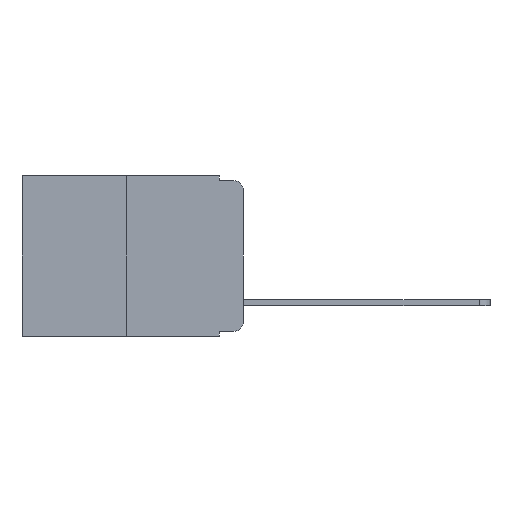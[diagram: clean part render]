
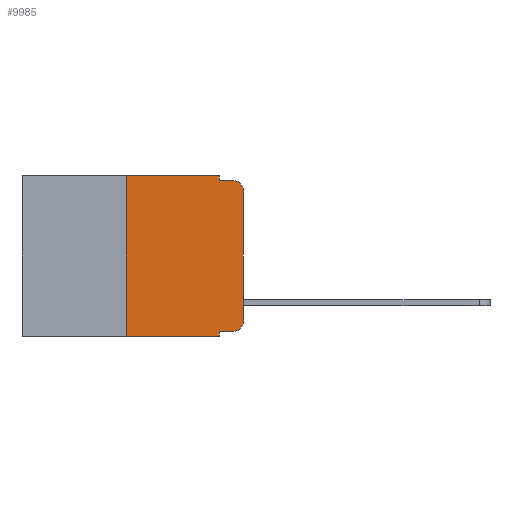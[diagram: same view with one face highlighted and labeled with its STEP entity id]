
A CAD part, left-side view. The second image highlights one B-rep face of the part: STEP entity #9985.
In plain terms, the highlighted planar face has unit normal (-1, 0, 0).
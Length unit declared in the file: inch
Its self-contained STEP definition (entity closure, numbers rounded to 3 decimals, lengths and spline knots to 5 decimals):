
#44 = EDGE_CURVE ( 'NONE', #7193, #5768, #9298, .T. ) ;
#143 = DIRECTION ( 'NONE',  ( 0., 0., -1. ) ) ;
#144 = DIRECTION ( 'NONE',  ( 1., 0., 0. ) ) ;
#146 = CARTESIAN_POINT ( 'NONE',  ( 0., 0.051, -0.333 ) ) ;
#195 = ORIENTED_EDGE ( 'NONE', *, *, #2460, .T. ) ;
#224 = ORIENTED_EDGE ( 'NONE', *, *, #729, .T. ) ;
#228 = ORIENTED_EDGE ( 'NONE', *, *, #5570, .T. ) ;
#243 = ORIENTED_EDGE ( 'NONE', *, *, #44, .F. ) ;
#250 = CARTESIAN_POINT ( 'NONE',  ( 0., 0.473, 0. ) ) ;
#254 = ORIENTED_EDGE ( 'NONE', *, *, #1778, .F. ) ;
#261 = PLANE ( 'NONE',  #674 ) ;
#286 = CARTESIAN_POINT ( 'NONE',  ( 0., 0.02, -0.01 ) ) ;
#310 = DIRECTION ( 'NONE',  ( 0., 0., -1. ) ) ;
#318 = ORIENTED_EDGE ( 'NONE', *, *, #6520, .F. ) ;
#331 = EDGE_CURVE ( 'NONE', #5768, #7864, #2317, .T. ) ;
#348 = ORIENTED_EDGE ( 'NONE', *, *, #866, .F. ) ;
#425 = ORIENTED_EDGE ( 'NONE', *, *, #331, .F. ) ;
#511 = VECTOR ( 'NONE', #8199, 39.37008 ) ;
#674 = AXIS2_PLACEMENT_3D ( 'NONE', #250, #144, #143 ) ;
#729 = EDGE_CURVE ( 'NONE', #6188, #8211, #9358, .T. ) ;
#771 = VERTEX_POINT ( 'NONE', #4075 ) ;
#786 = AXIS2_PLACEMENT_3D ( 'NONE', #5343, #2630, #2617 ) ;
#866 = EDGE_CURVE ( 'NONE', #5657, #8211, #4388, .T. ) ;
#964 = ORIENTED_EDGE ( 'NONE', *, *, #8743, .T. ) ;
#1014 = ORIENTED_EDGE ( 'NONE', *, *, #2843, .T. ) ;
#1099 = DIRECTION ( 'NONE',  ( 0., 0., -1. ) ) ;
#1351 = FACE_OUTER_BOUND ( 'NONE', #4818, .T. ) ;
#1778 = EDGE_CURVE ( 'NONE', #771, #3837, #5374, .T. ) ;
#1902 = CARTESIAN_POINT ( 'NONE',  ( 0., 0., 0. ) ) ;
#2183 = CARTESIAN_POINT ( 'NONE',  ( 0., 0.473, 0. ) ) ;
#2317 = LINE ( 'NONE', #2183, #6264 ) ;
#2460 = EDGE_CURVE ( 'NONE', #3702, #6188, #8965, .T. ) ;
#2617 = DIRECTION ( 'NONE',  ( 0., 0., -1. ) ) ;
#2630 = DIRECTION ( 'NONE',  ( -1., 0., 0. ) ) ;
#2804 = CARTESIAN_POINT ( 'NONE',  ( 0., 0.473, -0.343 ) ) ;
#2843 = EDGE_CURVE ( 'NONE', #771, #7341, #9427, .T. ) ;
#2847 = DIRECTION ( 'NONE',  ( 0., -1., 0. ) ) ;
#2858 = VECTOR ( 'NONE', #4511, 39.37008 ) ;
#2960 = VECTOR ( 'NONE', #8017, 39.37008 ) ;
#2998 = VECTOR ( 'NONE', #1099, 39.37008 ) ;
#3281 = VECTOR ( 'NONE', #310, 39.37008 ) ;
#3545 = CARTESIAN_POINT ( 'NONE',  ( 0., 0., -0.03 ) ) ;
#3603 = CIRCLE ( 'NONE', #4490, 0.02 ) ;
#3702 = VERTEX_POINT ( 'NONE', #5370 ) ;
#3837 = VERTEX_POINT ( 'NONE', #3877 ) ;
#3877 = CARTESIAN_POINT ( 'NONE',  ( 0., 0.051, -0.343 ) ) ;
#3933 = CARTESIAN_POINT ( 'NONE',  ( 0., 0.051, -0.01 ) ) ;
#4075 = CARTESIAN_POINT ( 'NONE',  ( 0., 0.051, -0.333 ) ) ;
#4388 = LINE ( 'NONE', #3933, #8197 ) ;
#4490 = AXIS2_PLACEMENT_3D ( 'NONE', #8316, #8260, #7476 ) ;
#4511 = DIRECTION ( 'NONE',  ( 0., 0., 1. ) ) ;
#4594 = CARTESIAN_POINT ( 'NONE',  ( 0., 0.051, 0. ) ) ;
#4690 = LINE ( 'NONE', #2804, #511 ) ;
#4727 = CARTESIAN_POINT ( 'NONE',  ( 0., 0.25, -0.343 ) ) ;
#4818 = EDGE_LOOP ( 'NONE', ( #195, #224, #348, #318, #425, #243, #228, #254, #1014, #964 ) ) ;
#5011 = CARTESIAN_POINT ( 'NONE',  ( 0., 0.02, -0.333 ) ) ;
#5155 = LINE ( 'NONE', #6027, #3281 ) ;
#5343 = CARTESIAN_POINT ( 'NONE',  ( 0., 0.02, -0.03 ) ) ;
#5370 = CARTESIAN_POINT ( 'NONE',  ( 0., 0., -0.313 ) ) ;
#5374 = LINE ( 'NONE', #7555, #2998 ) ;
#5570 = EDGE_CURVE ( 'NONE', #7193, #3837, #4690, .T. ) ;
#5657 = VERTEX_POINT ( 'NONE', #7430 ) ;
#5768 = VERTEX_POINT ( 'NONE', #8008 ) ;
#6027 = CARTESIAN_POINT ( 'NONE',  ( 0., 0.051, 0. ) ) ;
#6188 = VERTEX_POINT ( 'NONE', #3545 ) ;
#6264 = VECTOR ( 'NONE', #2847, 39.37008 ) ;
#6520 = EDGE_CURVE ( 'NONE', #7864, #5657, #5155, .T. ) ;
#6800 = DIRECTION ( 'NONE',  ( 0., -1., 0. ) ) ;
#7193 = VERTEX_POINT ( 'NONE', #4727 ) ;
#7341 = VERTEX_POINT ( 'NONE', #5011 ) ;
#7427 = CARTESIAN_POINT ( 'NONE',  ( 0., 0.25, 0. ) ) ;
#7430 = CARTESIAN_POINT ( 'NONE',  ( 0., 0.051, -0.01 ) ) ;
#7471 = VECTOR ( 'NONE', #9579, 39.37008 ) ;
#7476 = DIRECTION ( 'NONE',  ( 0., 0., -1. ) ) ;
#7555 = CARTESIAN_POINT ( 'NONE',  ( 0., 0.051, 0. ) ) ;
#7864 = VERTEX_POINT ( 'NONE', #4594 ) ;
#8008 = CARTESIAN_POINT ( 'NONE',  ( 0., 0.25, 0. ) ) ;
#8017 = DIRECTION ( 'NONE',  ( 0., 0., 1. ) ) ;
#8197 = VECTOR ( 'NONE', #6800, 39.37008 ) ;
#8199 = DIRECTION ( 'NONE',  ( 0., -1., 0. ) ) ;
#8211 = VERTEX_POINT ( 'NONE', #286 ) ;
#8260 = DIRECTION ( 'NONE',  ( -1., 0., 0. ) ) ;
#8316 = CARTESIAN_POINT ( 'NONE',  ( 0., 0.02, -0.313 ) ) ;
#8743 = EDGE_CURVE ( 'NONE', #7341, #3702, #3603, .T. ) ;
#8965 = LINE ( 'NONE', #1902, #2858 ) ;
#9298 = LINE ( 'NONE', #7427, #2960 ) ;
#9358 = CIRCLE ( 'NONE', #786, 0.02 ) ;
#9427 = LINE ( 'NONE', #146, #7471 ) ;
#9579 = DIRECTION ( 'NONE',  ( 0., -1., 0. ) ) ;
#9985 = ADVANCED_FACE ( 'NONE', ( #1351 ), #261, .F. ) ;
